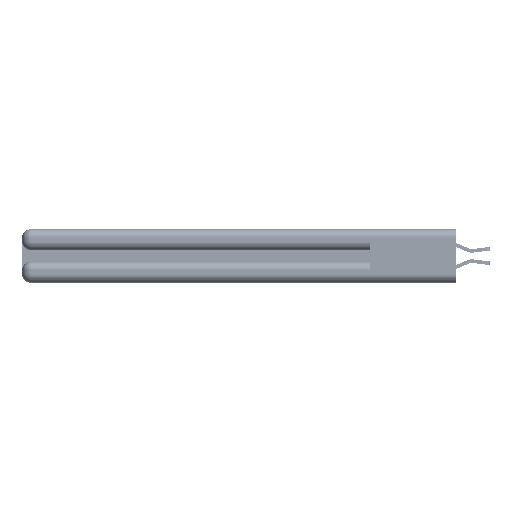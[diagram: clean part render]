
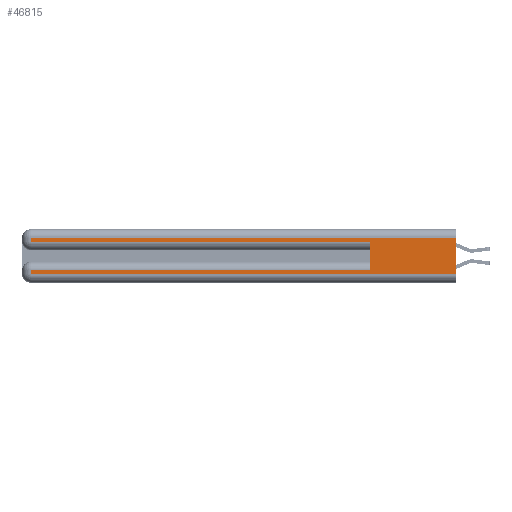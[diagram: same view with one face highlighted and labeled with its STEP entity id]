
A CAD part, left-side view. The second image highlights one B-rep face of the part: STEP entity #46815.
In plain terms, the highlighted planar face has unit normal (-1, 0, 0).
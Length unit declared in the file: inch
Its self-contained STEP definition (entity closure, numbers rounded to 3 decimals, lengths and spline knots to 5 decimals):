
#1162 = DIRECTION ( 'NONE',  ( 0., 1., 0. ) ) ;
#1226 = ORIENTED_EDGE ( 'NONE', *, *, #46680, .T. ) ;
#2593 = VECTOR ( 'NONE', #3445, 39.37008 ) ;
#3333 = VECTOR ( 'NONE', #7008, 39.37008 ) ;
#3348 = CARTESIAN_POINT ( 'NONE',  ( 0., 0., 0.06 ) ) ;
#3445 = DIRECTION ( 'NONE',  ( 0., -1., 0. ) ) ;
#4048 = AXIS2_PLACEMENT_3D ( 'NONE', #23607, #12069, #39581 ) ;
#4660 = ORIENTED_EDGE ( 'NONE', *, *, #17486, .F. ) ;
#5617 = VERTEX_POINT ( 'NONE', #7255 ) ;
#6687 = CARTESIAN_POINT ( 'NONE',  ( 0., 0., 0.06 ) ) ;
#7008 = DIRECTION ( 'NONE',  ( 0., 0., -1. ) ) ;
#7255 = CARTESIAN_POINT ( 'NONE',  ( 0., 0., 0.31 ) ) ;
#8072 = PLANE ( 'NONE',  #4048 ) ;
#8418 = CARTESIAN_POINT ( 'NONE',  ( 0., 2.94, 0.37 ) ) ;
#8441 = VECTOR ( 'NONE', #1162, 39.37008 ) ;
#9019 = VERTEX_POINT ( 'NONE', #31981 ) ;
#9112 = ORIENTED_EDGE ( 'NONE', *, *, #43597, .T. ) ;
#9669 = LINE ( 'NONE', #36461, #8441 ) ;
#9926 = CARTESIAN_POINT ( 'NONE',  ( 0., 2.94, 0.085 ) ) ;
#10896 = ORIENTED_EDGE ( 'NONE', *, *, #50272, .T. ) ;
#11256 = ORIENTED_EDGE ( 'NONE', *, *, #27119, .T. ) ;
#11783 = LINE ( 'NONE', #3348, #21054 ) ;
#11974 = VERTEX_POINT ( 'NONE', #6687 ) ;
#12069 = DIRECTION ( 'NONE',  ( 1., 0., 0. ) ) ;
#13057 = LINE ( 'NONE', #46618, #2593 ) ;
#13323 = EDGE_LOOP ( 'NONE', ( #44373, #49122, #45821, #1226, #4660, #9112, #10896, #11256 ) ) ;
#16042 = DIRECTION ( 'NONE',  ( 0., 1., 0. ) ) ;
#17486 = EDGE_CURVE ( 'NONE', #44777, #32224, #21681, .T. ) ;
#18080 = CARTESIAN_POINT ( 'NONE',  ( 0., 0., 0.37 ) ) ;
#20894 = LINE ( 'NONE', #47461, #31373 ) ;
#21054 = VECTOR ( 'NONE', #34889, 39.37008 ) ;
#21681 = LINE ( 'NONE', #48439, #33420 ) ;
#23607 = CARTESIAN_POINT ( 'NONE',  ( 0., 0., 0.37 ) ) ;
#24941 = DIRECTION ( 'NONE',  ( 0., 0., 1. ) ) ;
#25556 = LINE ( 'NONE', #34610, #3333 ) ;
#25667 = CARTESIAN_POINT ( 'NONE',  ( 0., 2.94, 0.06 ) ) ;
#27119 = EDGE_CURVE ( 'NONE', #37462, #11974, #11783, .T. ) ;
#31373 = VECTOR ( 'NONE', #16042, 39.37008 ) ;
#31541 = VECTOR ( 'NONE', #36014, 39.37008 ) ;
#31981 = CARTESIAN_POINT ( 'NONE',  ( 0., 2.94, 0.31 ) ) ;
#32224 = VERTEX_POINT ( 'NONE', #43412 ) ;
#33420 = VECTOR ( 'NONE', #24941, 39.37008 ) ;
#33687 = VECTOR ( 'NONE', #47029, 39.37008 ) ;
#34238 = EDGE_CURVE ( 'NONE', #5617, #11974, #34897, .T. ) ;
#34610 = CARTESIAN_POINT ( 'NONE',  ( 0., 2.94, 0.37 ) ) ;
#34889 = DIRECTION ( 'NONE',  ( 0., -1., 0. ) ) ;
#34897 = LINE ( 'NONE', #18080, #33687 ) ;
#35457 = EDGE_CURVE ( 'NONE', #9019, #38658, #25556, .T. ) ;
#36014 = DIRECTION ( 'NONE',  ( 0., 0., -1. ) ) ;
#36461 = CARTESIAN_POINT ( 'NONE',  ( 0., 0., 0.085 ) ) ;
#37078 = FACE_OUTER_BOUND ( 'NONE', #13323, .T. ) ;
#37462 = VERTEX_POINT ( 'NONE', #25667 ) ;
#38658 = VERTEX_POINT ( 'NONE', #41153 ) ;
#39581 = DIRECTION ( 'NONE',  ( 0., 0., -1. ) ) ;
#40692 = LINE ( 'NONE', #8418, #31541 ) ;
#41153 = CARTESIAN_POINT ( 'NONE',  ( 0., 2.94, 0.285 ) ) ;
#42835 = EDGE_CURVE ( 'NONE', #5617, #9019, #20894, .T. ) ;
#42988 = CARTESIAN_POINT ( 'NONE',  ( 0., 0.6, 0.085 ) ) ;
#43412 = CARTESIAN_POINT ( 'NONE',  ( 0., 0.6, 0.285 ) ) ;
#43597 = EDGE_CURVE ( 'NONE', #44777, #50756, #9669, .T. ) ;
#44373 = ORIENTED_EDGE ( 'NONE', *, *, #34238, .F. ) ;
#44777 = VERTEX_POINT ( 'NONE', #42988 ) ;
#45821 = ORIENTED_EDGE ( 'NONE', *, *, #35457, .T. ) ;
#46618 = CARTESIAN_POINT ( 'NONE',  ( 0., 0., 0.285 ) ) ;
#46680 = EDGE_CURVE ( 'NONE', #38658, #32224, #13057, .T. ) ;
#46815 = ADVANCED_FACE ( 'NONE', ( #37078 ), #8072, .F. ) ;
#47029 = DIRECTION ( 'NONE',  ( 0., 0., -1. ) ) ;
#47461 = CARTESIAN_POINT ( 'NONE',  ( 0., 0., 0.31 ) ) ;
#48439 = CARTESIAN_POINT ( 'NONE',  ( 0., 0.6, 0.145 ) ) ;
#49122 = ORIENTED_EDGE ( 'NONE', *, *, #42835, .T. ) ;
#50272 = EDGE_CURVE ( 'NONE', #50756, #37462, #40692, .T. ) ;
#50756 = VERTEX_POINT ( 'NONE', #9926 ) ;
